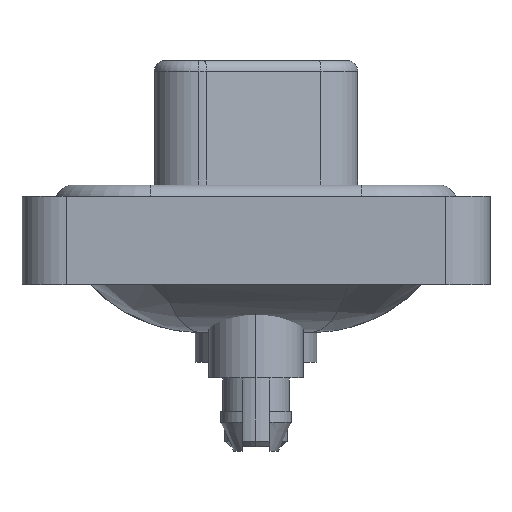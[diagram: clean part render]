
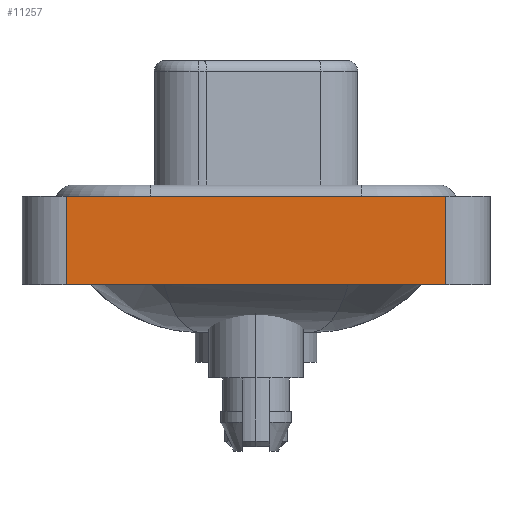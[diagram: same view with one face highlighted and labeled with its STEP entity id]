
A CAD part, left-side view. The second image highlights one B-rep face of the part: STEP entity #11257.
In plain terms, the highlighted planar face has unit normal (-1, 0, 0).
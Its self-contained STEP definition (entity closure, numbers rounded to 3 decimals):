
#391 = LINE ( 'NONE', #13923, #15732 ) ;
#899 = CARTESIAN_POINT ( 'NONE',  ( -7.25, 8.55, -3.6 ) ) ;
#1647 = ORIENTED_EDGE ( 'NONE', *, *, #13149, .T. ) ;
#1995 = DIRECTION ( 'NONE',  ( 0., 0., 1. ) ) ;
#2252 = LINE ( 'NONE', #13198, #2371 ) ;
#2371 = VECTOR ( 'NONE', #7252, 1000. ) ;
#2608 = VERTEX_POINT ( 'NONE', #899 ) ;
#2987 = EDGE_CURVE ( 'NONE', #9753, #5834, #2252, .T. ) ;
#3484 = LINE ( 'NONE', #9608, #12794 ) ;
#3499 = AXIS2_PLACEMENT_3D ( 'NONE', #9415, #7754, #1995 ) ;
#3621 = ORIENTED_EDGE ( 'NONE', *, *, #9607, .F. ) ;
#5618 = DIRECTION ( 'NONE',  ( 0., -1., 0. ) ) ;
#5834 = VERTEX_POINT ( 'NONE', #12069 ) ;
#6106 = CARTESIAN_POINT ( 'NONE',  ( -7.25, 8.55, 0.4 ) ) ;
#7106 = DIRECTION ( 'NONE',  ( 0., -1., 0. ) ) ;
#7252 = DIRECTION ( 'NONE',  ( 0., 0., 1. ) ) ;
#7600 = VECTOR ( 'NONE', #14168, 1000. ) ;
#7754 = DIRECTION ( 'NONE',  ( -1., 0., 0. ) ) ;
#7829 = PLANE ( 'NONE',  #3499 ) ;
#7941 = EDGE_CURVE ( 'NONE', #9760, #5834, #391, .T. ) ;
#8135 = CARTESIAN_POINT ( 'NONE',  ( -7.25, 8.55, -3.6 ) ) ;
#8985 = EDGE_LOOP ( 'NONE', ( #11336, #15085, #3621, #1647 ) ) ;
#9415 = CARTESIAN_POINT ( 'NONE',  ( -7.25, -8.55, -3.6 ) ) ;
#9607 = EDGE_CURVE ( 'NONE', #2608, #9760, #15372, .T. ) ;
#9608 = CARTESIAN_POINT ( 'NONE',  ( -7.25, -8.55, -3.6 ) ) ;
#9753 = VERTEX_POINT ( 'NONE', #10322 ) ;
#9760 = VERTEX_POINT ( 'NONE', #6106 ) ;
#10322 = CARTESIAN_POINT ( 'NONE',  ( -7.25, -8.55, -3.6 ) ) ;
#11257 = ADVANCED_FACE ( 'NONE', ( #11371 ), #7829, .T. ) ;
#11336 = ORIENTED_EDGE ( 'NONE', *, *, #2987, .T. ) ;
#11371 = FACE_OUTER_BOUND ( 'NONE', #8985, .T. ) ;
#12069 = CARTESIAN_POINT ( 'NONE',  ( -7.25, -8.55, 0.4 ) ) ;
#12794 = VECTOR ( 'NONE', #7106, 1000. ) ;
#13149 = EDGE_CURVE ( 'NONE', #2608, #9753, #3484, .T. ) ;
#13198 = CARTESIAN_POINT ( 'NONE',  ( -7.25, -8.55, -3.6 ) ) ;
#13923 = CARTESIAN_POINT ( 'NONE',  ( -7.25, -8.55, 0.4 ) ) ;
#14168 = DIRECTION ( 'NONE',  ( 0., 0., 1. ) ) ;
#15085 = ORIENTED_EDGE ( 'NONE', *, *, #7941, .F. ) ;
#15372 = LINE ( 'NONE', #8135, #7600 ) ;
#15732 = VECTOR ( 'NONE', #5618, 1000. ) ;
